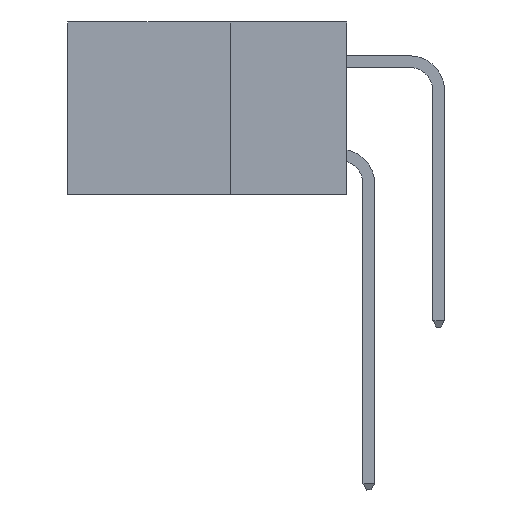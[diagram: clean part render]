
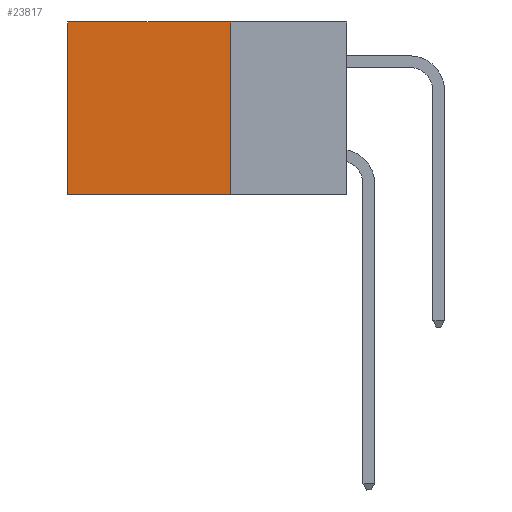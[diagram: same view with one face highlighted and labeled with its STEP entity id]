
A CAD part, left-side view. The second image highlights one B-rep face of the part: STEP entity #23817.
In plain terms, the highlighted planar face has unit normal (-1, 0, 0).
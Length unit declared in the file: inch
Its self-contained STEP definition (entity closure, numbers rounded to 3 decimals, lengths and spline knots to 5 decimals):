
#27 = VERTEX_POINT ( 'NONE', #21058 ) ;
#721 = VECTOR ( 'NONE', #8099, 39.37008 ) ;
#782 = EDGE_LOOP ( 'NONE', ( #5528, #29081, #9347, #9974 ) ) ;
#969 = FACE_OUTER_BOUND ( 'NONE', #782, .T. ) ;
#1268 = VERTEX_POINT ( 'NONE', #12698 ) ;
#1601 = VECTOR ( 'NONE', #31511, 39.37008 ) ;
#3050 = VECTOR ( 'NONE', #13842, 39.37008 ) ;
#3529 = DIRECTION ( 'NONE',  ( 0., 1., 0. ) ) ;
#5528 = ORIENTED_EDGE ( 'NONE', *, *, #14137, .T. ) ;
#6085 = CARTESIAN_POINT ( 'NONE',  ( 0.2875, 0.25, -0.37 ) ) ;
#6264 = DIRECTION ( 'NONE',  ( 0., 0., -1. ) ) ;
#8099 = DIRECTION ( 'NONE',  ( 0., 0., -1. ) ) ;
#8462 = EDGE_CURVE ( 'NONE', #9556, #27, #10668, .T. ) ;
#8664 = PLANE ( 'NONE',  #13055 ) ;
#9347 = ORIENTED_EDGE ( 'NONE', *, *, #33350, .F. ) ;
#9556 = VERTEX_POINT ( 'NONE', #12232 ) ;
#9974 = ORIENTED_EDGE ( 'NONE', *, *, #8462, .T. ) ;
#10668 = LINE ( 'NONE', #21096, #1601 ) ;
#12232 = CARTESIAN_POINT ( 'NONE',  ( 0.2875, 0.25, 0. ) ) ;
#12698 = CARTESIAN_POINT ( 'NONE',  ( 0.2875, 0.6, -0.37 ) ) ;
#13055 = AXIS2_PLACEMENT_3D ( 'NONE', #29682, #29518, #6264 ) ;
#13382 = VECTOR ( 'NONE', #3529, 39.37008 ) ;
#13496 = CARTESIAN_POINT ( 'NONE',  ( 0.2875, 0.25, 0. ) ) ;
#13842 = DIRECTION ( 'NONE',  ( 0., 0., -1. ) ) ;
#14137 = EDGE_CURVE ( 'NONE', #27, #1268, #16149, .T. ) ;
#16149 = LINE ( 'NONE', #26568, #721 ) ;
#16240 = LINE ( 'NONE', #13496, #3050 ) ;
#19081 = LINE ( 'NONE', #6085, #13382 ) ;
#21058 = CARTESIAN_POINT ( 'NONE',  ( 0.2875, 0.6, 0. ) ) ;
#21096 = CARTESIAN_POINT ( 'NONE',  ( 0.2875, 0.25, 0. ) ) ;
#23414 = CARTESIAN_POINT ( 'NONE',  ( 0.2875, 0.25, -0.37 ) ) ;
#23817 = ADVANCED_FACE ( 'NONE', ( #969 ), #8664, .F. ) ;
#26568 = CARTESIAN_POINT ( 'NONE',  ( 0.2875, 0.6, 0. ) ) ;
#29081 = ORIENTED_EDGE ( 'NONE', *, *, #32498, .F. ) ;
#29518 = DIRECTION ( 'NONE',  ( 1., 0., 0. ) ) ;
#29682 = CARTESIAN_POINT ( 'NONE',  ( 0.2875, 0.25, 0. ) ) ;
#30740 = VERTEX_POINT ( 'NONE', #23414 ) ;
#31511 = DIRECTION ( 'NONE',  ( 0., 1., 0. ) ) ;
#32498 = EDGE_CURVE ( 'NONE', #30740, #1268, #19081, .T. ) ;
#33350 = EDGE_CURVE ( 'NONE', #9556, #30740, #16240, .T. ) ;
